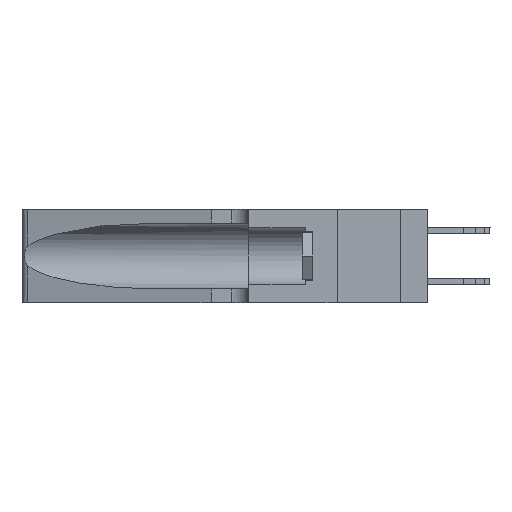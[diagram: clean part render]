
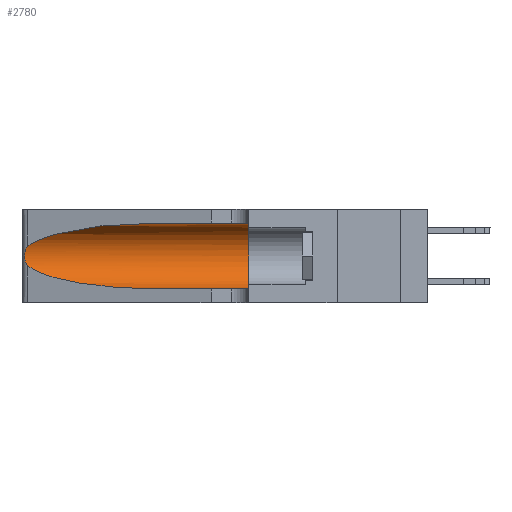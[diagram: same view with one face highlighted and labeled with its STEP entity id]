
A CAD part, left-side view. The second image highlights one B-rep face of the part: STEP entity #2780.
In plain terms, the highlighted cylindrical face has radius 3.308 mm (diameter 6.617 mm), a partial arc.
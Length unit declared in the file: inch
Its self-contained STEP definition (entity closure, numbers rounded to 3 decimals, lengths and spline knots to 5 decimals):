
#1466 = CARTESIAN_POINT ( 'NONE',  ( 0.18966, 0.96281, 0.05475 ) ) ;
#1690 = DIRECTION ( 'NONE',  ( 0., -1., 0. ) ) ;
#1955 = CARTESIAN_POINT ( 'NONE',  ( 0.25856, 1.23593, 0.16098 ) ) ;
#2047 = ORIENTED_EDGE ( 'NONE', *, *, #7352, .F. ) ;
#2188 = FACE_OUTER_BOUND ( 'NONE', #34981, .T. ) ;
#2780 = ADVANCED_FACE ( 'NONE', ( #2188 ), #23006, .F. ) ;
#4061 = CARTESIAN_POINT ( 'NONE',  ( 0.1305, 1.61858, 0.31525 ) ) ;
#4189 = CARTESIAN_POINT ( 'NONE',  ( 0.1305, 0.72297, 0.31525 ) ) ;
#4438 = EDGE_CURVE ( 'NONE', #33161, #12866, #20603, .T. ) ;
#5621 = DIRECTION ( 'NONE',  ( 0., -1., 0. ) ) ;
#6651 = CARTESIAN_POINT ( 'NONE',  ( 0.25487, 1.22718, 0.14631 ) ) ;
#6717 = VERTEX_POINT ( 'NONE', #31760 ) ;
#6734 = VECTOR ( 'NONE', #15166, 39.37008 ) ;
#7013 = CARTESIAN_POINT ( 'NONE',  ( 0.2373, 1.15595, 0.28018 ) ) ;
#7352 = EDGE_CURVE ( 'NONE', #33161, #30996, #11949, .T. ) ;
#7874 = CARTESIAN_POINT ( 'NONE',  ( 0.26075, 1.23896, 0.178 ) ) ;
#8674 = CARTESIAN_POINT ( 'NONE',  ( 0.1305, 0.35, 0.185 ) ) ;
#10057 = CARTESIAN_POINT ( 'NONE',  ( 0.1305, 0.72297, 0.31525 ) ) ;
#10173 = CARTESIAN_POINT ( 'NONE',  ( 0.26075, 1.23896, 0.19203 ) ) ;
#10618 = ORIENTED_EDGE ( 'NONE', *, *, #14866, .T. ) ;
#10776 = ORIENTED_EDGE ( 'NONE', *, *, #20017, .T. ) ;
#11415 = AXIS2_PLACEMENT_3D ( 'NONE', #27295, #5621, #24993 ) ;
#11949 = LINE ( 'NONE', #4061, #6734 ) ;
#12866 = VERTEX_POINT ( 'NONE', #26989 ) ;
#13440 = CARTESIAN_POINT ( 'NONE',  ( 0.25854, 1.2359, 0.20912 ) ) ;
#14866 = EDGE_CURVE ( 'NONE', #12866, #24965, #24392, .T. ) ;
#15166 = DIRECTION ( 'NONE',  ( 0., -1., 0. ) ) ;
#15719 = VERTEX_POINT ( 'NONE', #28989 ) ;
#15964 = CARTESIAN_POINT ( 'NONE',  ( 0.26017, 1.23833, 0.17102 ) ) ;
#16091 = CARTESIAN_POINT ( 'NONE',  ( 0.25487, 1.22718, 0.14631 ) ) ;
#18124 = ORIENTED_EDGE ( 'NONE', *, *, #19357, .T. ) ;
#19035 = CARTESIAN_POINT ( 'NONE',  ( 0.1305, 0.72297, 0.05475 ) ) ;
#19357 = EDGE_CURVE ( 'NONE', #24965, #6717, #21530, .T. ) ;
#20017 = EDGE_CURVE ( 'NONE', #6717, #15719, #29002, .T. ) ;
#20603 =( BOUNDED_CURVE ( )  B_SPLINE_CURVE ( 3, ( #10057, #23904, #7013, #26279 ),
 .UNSPECIFIED., .F., .F. ) 
 B_SPLINE_CURVE_WITH_KNOTS ( ( 4, 4 ),
 ( 1.5708, 2.84003 ),
 .UNSPECIFIED. ) 
 CURVE ( )  GEOMETRIC_REPRESENTATION_ITEM ( )  RATIONAL_B_SPLINE_CURVE ( ( 1., 0.87, 0.87, 1. ) ) 
 REPRESENTATION_ITEM ( '' )  );
#21458 = CARTESIAN_POINT ( 'NONE',  ( 0.26018, 1.23835, 0.19895 ) ) ;
#21530 =( BOUNDED_CURVE ( )  B_SPLINE_CURVE ( 3, ( #35645, #24622, #1466, #19035 ),
 .UNSPECIFIED., .F., .T. ) 
 B_SPLINE_CURVE_WITH_KNOTS ( ( 4, 4 ),
 ( 3.44316, 4.71239 ),
 .UNSPECIFIED. ) 
 CURVE ( )  GEOMETRIC_REPRESENTATION_ITEM ( )  RATIONAL_B_SPLINE_CURVE ( ( 1., 0.87, 0.87, 1. ) ) 
 REPRESENTATION_ITEM ( '' )  );
#21560 = EDGE_CURVE ( 'NONE', #30996, #15719, #34110, .T. ) ;
#23006 = CYLINDRICAL_SURFACE ( 'NONE', #11415, 0.13025 ) ;
#23655 = CARTESIAN_POINT ( 'NONE',  ( 0.25487, 1.22718, 0.22369 ) ) ;
#23904 = CARTESIAN_POINT ( 'NONE',  ( 0.18966, 0.96281, 0.31525 ) ) ;
#24392 = B_SPLINE_CURVE_WITH_KNOTS ( 'NONE', 3,
 ( #23655, #34758, #32113, #32591, #13440, #21458, #10173, #7874, #15964, #1955, #35388, #32833, #27239, #16091 ),
 .UNSPECIFIED., .F., .F.,
 ( 4, 2, 2, 2, 2, 2, 4 ),
 ( 0., 0.00027, 0.00053, 0.00107, 0.0016, 0.00187, 0.00214 ),
 .UNSPECIFIED. ) ;
#24622 = CARTESIAN_POINT ( 'NONE',  ( 0.2373, 1.15595, 0.08982 ) ) ;
#24965 = VERTEX_POINT ( 'NONE', #6651 ) ;
#24993 = DIRECTION ( 'NONE',  ( 0., 0., -1. ) ) ;
#26279 = CARTESIAN_POINT ( 'NONE',  ( 0.25487, 1.22718, 0.22369 ) ) ;
#26989 = CARTESIAN_POINT ( 'NONE',  ( 0.25487, 1.22718, 0.22369 ) ) ;
#27239 = CARTESIAN_POINT ( 'NONE',  ( 0.25555, 1.22993, 0.14849 ) ) ;
#27295 = CARTESIAN_POINT ( 'NONE',  ( 0.1305, 1.61858, 0.185 ) ) ;
#27461 = CARTESIAN_POINT ( 'NONE',  ( 0.1305, 0.35, 0.31525 ) ) ;
#28040 = DIRECTION ( 'NONE',  ( 0., 1., 0. ) ) ;
#28989 = CARTESIAN_POINT ( 'NONE',  ( 0.1305, 0.35, 0.05475 ) ) ;
#29002 = LINE ( 'NONE', #34860, #30760 ) ;
#29077 = AXIS2_PLACEMENT_3D ( 'NONE', #8674, #28040, #31189 ) ;
#30314 = ORIENTED_EDGE ( 'NONE', *, *, #21560, .F. ) ;
#30760 = VECTOR ( 'NONE', #1690, 39.37008 ) ;
#30996 = VERTEX_POINT ( 'NONE', #27461 ) ;
#31189 = DIRECTION ( 'NONE',  ( 0., 0., 1. ) ) ;
#31760 = CARTESIAN_POINT ( 'NONE',  ( 0.1305, 0.72297, 0.05475 ) ) ;
#32113 = CARTESIAN_POINT ( 'NONE',  ( 0.25639, 1.23184, 0.21858 ) ) ;
#32591 = CARTESIAN_POINT ( 'NONE',  ( 0.25787, 1.23484, 0.2124 ) ) ;
#32833 = CARTESIAN_POINT ( 'NONE',  ( 0.25639, 1.23186, 0.15144 ) ) ;
#33161 = VERTEX_POINT ( 'NONE', #4189 ) ;
#34110 = CIRCLE ( 'NONE', #29077, 0.13025 ) ;
#34221 = ORIENTED_EDGE ( 'NONE', *, *, #4438, .T. ) ;
#34758 = CARTESIAN_POINT ( 'NONE',  ( 0.25555, 1.22994, 0.2215 ) ) ;
#34860 = CARTESIAN_POINT ( 'NONE',  ( 0.1305, 1.61858, 0.05475 ) ) ;
#34981 = EDGE_LOOP ( 'NONE', ( #34221, #10618, #18124, #10776, #30314, #2047 ) ) ;
#35388 = CARTESIAN_POINT ( 'NONE',  ( 0.25789, 1.23486, 0.15765 ) ) ;
#35645 = CARTESIAN_POINT ( 'NONE',  ( 0.25487, 1.22718, 0.14631 ) ) ;
